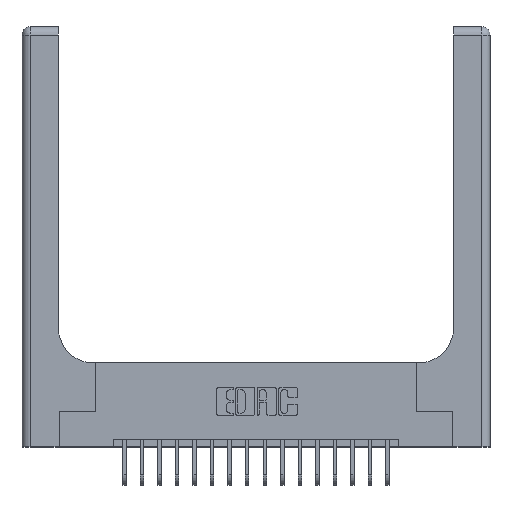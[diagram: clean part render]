
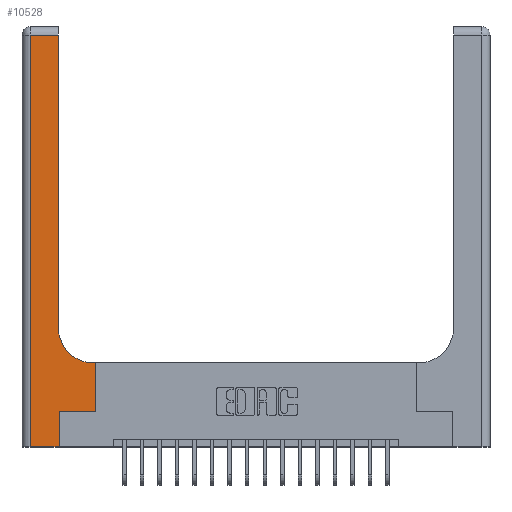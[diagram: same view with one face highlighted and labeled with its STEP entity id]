
A CAD part, top view. The second image highlights one B-rep face of the part: STEP entity #10528.
In plain terms, the highlighted planar face has unit normal (0, 0, 1).
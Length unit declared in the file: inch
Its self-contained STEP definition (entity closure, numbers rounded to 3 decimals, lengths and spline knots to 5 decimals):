
#492 = CARTESIAN_POINT ( 'NONE',  ( 0.265, 0., 0.37 ) ) ;
#632 = DIRECTION ( 'NONE',  ( 0., 1., 0. ) ) ;
#805 = CARTESIAN_POINT ( 'NONE',  ( 0.265, 0.25, 0.37 ) ) ;
#821 = EDGE_CURVE ( 'NONE', #4949, #7597, #15038, .T. ) ;
#1122 = EDGE_CURVE ( 'NONE', #17791, #3752, #20412, .T. ) ;
#1242 = AXIS2_PLACEMENT_3D ( 'NONE', #13131, #1956, #16401 ) ;
#1888 = PLANE ( 'NONE',  #1242 ) ;
#1956 = DIRECTION ( 'NONE',  ( 0., 0., -1. ) ) ;
#2288 = CARTESIAN_POINT ( 'NONE',  ( 0.528, 0.25, 0.37 ) ) ;
#2371 = LINE ( 'NONE', #2288, #20078 ) ;
#2592 = CARTESIAN_POINT ( 'NONE',  ( 0.265, 0.25, 0.37 ) ) ;
#2809 = CARTESIAN_POINT ( 'NONE',  ( 0., 2.94, 0.37 ) ) ;
#2944 = VECTOR ( 'NONE', #18221, 39.37008 ) ;
#3305 = VERTEX_POINT ( 'NONE', #18492 ) ;
#3580 = VECTOR ( 'NONE', #13766, 39.37008 ) ;
#3687 = VERTEX_POINT ( 'NONE', #12943 ) ;
#3752 = VERTEX_POINT ( 'NONE', #13789 ) ;
#4949 = VERTEX_POINT ( 'NONE', #13113 ) ;
#5763 = CARTESIAN_POINT ( 'NONE',  ( 0.06, 2.94, 0.37 ) ) ;
#5897 = ORIENTED_EDGE ( 'NONE', *, *, #13677, .T. ) ;
#6021 = LINE ( 'NONE', #2809, #15355 ) ;
#6345 = CARTESIAN_POINT ( 'NONE',  ( 0.265, 0., 0.37 ) ) ;
#7149 = DIRECTION ( 'NONE',  ( 1., 0., 0. ) ) ;
#7163 = CARTESIAN_POINT ( 'NONE',  ( 0., 0., 0.37 ) ) ;
#7581 = DIRECTION ( 'NONE',  ( 0., 1., 0. ) ) ;
#7597 = VERTEX_POINT ( 'NONE', #6345 ) ;
#7961 = LINE ( 'NONE', #8485, #8720 ) ;
#8287 = FACE_OUTER_BOUND ( 'NONE', #15822, .T. ) ;
#8485 = CARTESIAN_POINT ( 'NONE',  ( 0.26, 0.6, 0.37 ) ) ;
#8501 = AXIS2_PLACEMENT_3D ( 'NONE', #20112, #10523, #7149 ) ;
#8720 = VECTOR ( 'NONE', #16667, 39.37008 ) ;
#8765 = ORIENTED_EDGE ( 'NONE', *, *, #16026, .T. ) ;
#9207 = CIRCLE ( 'NONE', #8501, 0.25 ) ;
#10196 = EDGE_CURVE ( 'NONE', #3752, #17344, #6021, .T. ) ;
#10322 = ORIENTED_EDGE ( 'NONE', *, *, #821, .T. ) ;
#10523 = DIRECTION ( 'NONE',  ( 0., 0., -1. ) ) ;
#10528 = ADVANCED_FACE ( 'NONE', ( #8287 ), #1888, .F. ) ;
#10875 = VECTOR ( 'NONE', #632, 39.37008 ) ;
#10933 = ORIENTED_EDGE ( 'NONE', *, *, #19760, .T. ) ;
#11045 = DIRECTION ( 'NONE',  ( -1., 0., 0. ) ) ;
#12198 = DIRECTION ( 'NONE',  ( 0., 1., 0. ) ) ;
#12943 = CARTESIAN_POINT ( 'NONE',  ( 0.528, 0.6, 0.37 ) ) ;
#13113 = CARTESIAN_POINT ( 'NONE',  ( 0.06, 0., 0.37 ) ) ;
#13131 = CARTESIAN_POINT ( 'NONE',  ( 0., 3., 0.37 ) ) ;
#13184 = VECTOR ( 'NONE', #18765, 39.37008 ) ;
#13452 = CARTESIAN_POINT ( 'NONE',  ( 0.26, 0.85, 0.37 ) ) ;
#13458 = ORIENTED_EDGE ( 'NONE', *, *, #17951, .T. ) ;
#13677 = EDGE_CURVE ( 'NONE', #3305, #17791, #9207, .T. ) ;
#13766 = DIRECTION ( 'NONE',  ( 1., 0., 0. ) ) ;
#13789 = CARTESIAN_POINT ( 'NONE',  ( 0.26, 2.94, 0.37 ) ) ;
#14669 = LINE ( 'NONE', #492, #10875 ) ;
#14733 = ORIENTED_EDGE ( 'NONE', *, *, #1122, .T. ) ;
#15038 = LINE ( 'NONE', #7163, #2944 ) ;
#15220 = VERTEX_POINT ( 'NONE', #17637 ) ;
#15355 = VECTOR ( 'NONE', #11045, 39.37008 ) ;
#15635 = ORIENTED_EDGE ( 'NONE', *, *, #10196, .T. ) ;
#15737 = LINE ( 'NONE', #20646, #13184 ) ;
#15822 = EDGE_LOOP ( 'NONE', ( #14733, #15635, #15936, #10322, #16109, #10933, #13458, #8765, #5897 ) ) ;
#15927 = LINE ( 'NONE', #2592, #3580 ) ;
#15936 = ORIENTED_EDGE ( 'NONE', *, *, #18109, .T. ) ;
#16026 = EDGE_CURVE ( 'NONE', #3687, #3305, #7961, .T. ) ;
#16109 = ORIENTED_EDGE ( 'NONE', *, *, #19547, .T. ) ;
#16401 = DIRECTION ( 'NONE',  ( -1., 0., 0. ) ) ;
#16667 = DIRECTION ( 'NONE',  ( -1., 0., 0. ) ) ;
#17344 = VERTEX_POINT ( 'NONE', #5763 ) ;
#17637 = CARTESIAN_POINT ( 'NONE',  ( 0.528, 0.25, 0.37 ) ) ;
#17791 = VERTEX_POINT ( 'NONE', #13452 ) ;
#17951 = EDGE_CURVE ( 'NONE', #15220, #3687, #2371, .T. ) ;
#18109 = EDGE_CURVE ( 'NONE', #17344, #4949, #15737, .T. ) ;
#18116 = VECTOR ( 'NONE', #7581, 39.37008 ) ;
#18221 = DIRECTION ( 'NONE',  ( 1., 0., 0. ) ) ;
#18492 = CARTESIAN_POINT ( 'NONE',  ( 0.51, 0.6, 0.37 ) ) ;
#18765 = DIRECTION ( 'NONE',  ( 0., -1., 0. ) ) ;
#18876 = VERTEX_POINT ( 'NONE', #805 ) ;
#18992 = CARTESIAN_POINT ( 'NONE',  ( 0.26, 3., 0.37 ) ) ;
#19547 = EDGE_CURVE ( 'NONE', #7597, #18876, #14669, .T. ) ;
#19760 = EDGE_CURVE ( 'NONE', #18876, #15220, #15927, .T. ) ;
#20078 = VECTOR ( 'NONE', #12198, 39.37008 ) ;
#20112 = CARTESIAN_POINT ( 'NONE',  ( 0.51, 0.85, 0.37 ) ) ;
#20412 = LINE ( 'NONE', #18992, #18116 ) ;
#20646 = CARTESIAN_POINT ( 'NONE',  ( 0.06, 3., 0.37 ) ) ;
